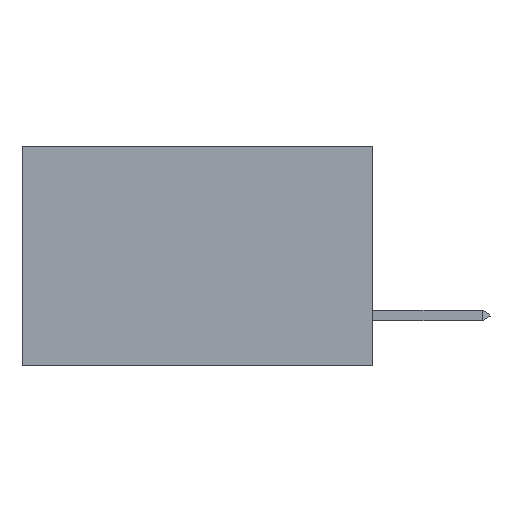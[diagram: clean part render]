
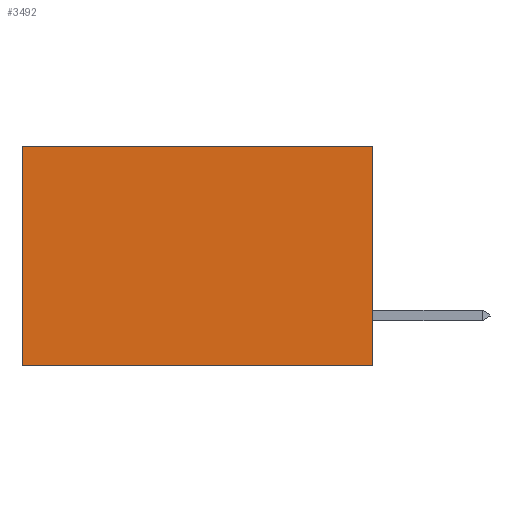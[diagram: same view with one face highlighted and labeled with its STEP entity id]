
A CAD part, left-side view. The second image highlights one B-rep face of the part: STEP entity #3492.
In plain terms, the highlighted planar face has unit normal (-1, 0, 0).
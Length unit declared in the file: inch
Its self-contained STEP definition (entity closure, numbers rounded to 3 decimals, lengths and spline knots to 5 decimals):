
#124 = ORIENTED_EDGE ( 'NONE', *, *, #6006, .F. ) ;
#918 = CARTESIAN_POINT ( 'NONE',  ( 0.277, 0.59, -0.37 ) ) ;
#1590 = CARTESIAN_POINT ( 'NONE',  ( 0.277, 0.59, -0.37 ) ) ;
#1830 = VECTOR ( 'NONE', #7440, 39.37008 ) ;
#2475 = CARTESIAN_POINT ( 'NONE',  ( 0.277, 0., 0. ) ) ;
#2851 = DIRECTION ( 'NONE',  ( 0., 0., -1. ) ) ;
#2853 = CARTESIAN_POINT ( 'NONE',  ( 0.277, 0., -0.37 ) ) ;
#3228 = LINE ( 'NONE', #1590, #7750 ) ;
#3387 = CARTESIAN_POINT ( 'NONE',  ( 0.277, 0., -0.37 ) ) ;
#3444 = PLANE ( 'NONE',  #10667 ) ;
#3492 = ADVANCED_FACE ( 'NONE', ( #8694 ), #3444, .F. ) ;
#3501 = DIRECTION ( 'NONE',  ( 0., 0., -1. ) ) ;
#3545 = DIRECTION ( 'NONE',  ( 1., 0., 0. ) ) ;
#5520 = ORIENTED_EDGE ( 'NONE', *, *, #8481, .F. ) ;
#5745 = ORIENTED_EDGE ( 'NONE', *, *, #10994, .T. ) ;
#5867 = CARTESIAN_POINT ( 'NONE',  ( 0.277, 0.59, 0. ) ) ;
#6006 = EDGE_CURVE ( 'NONE', #10157, #7099, #7083, .T. ) ;
#6203 = DIRECTION ( 'NONE',  ( 0., 0., -1. ) ) ;
#6572 = CARTESIAN_POINT ( 'NONE',  ( 0.277, 0., 0. ) ) ;
#7083 = LINE ( 'NONE', #2853, #8180 ) ;
#7099 = VERTEX_POINT ( 'NONE', #9924 ) ;
#7440 = DIRECTION ( 'NONE',  ( 0., 1., 0. ) ) ;
#7674 = CARTESIAN_POINT ( 'NONE',  ( 0.277, 0., -0.37 ) ) ;
#7750 = VECTOR ( 'NONE', #6203, 39.37008 ) ;
#7844 = VERTEX_POINT ( 'NONE', #5867 ) ;
#8180 = VECTOR ( 'NONE', #2851, 39.37008 ) ;
#8304 = VECTOR ( 'NONE', #9722, 39.37008 ) ;
#8481 = EDGE_CURVE ( 'NONE', #7099, #10109, #9129, .T. ) ;
#8608 = LINE ( 'NONE', #2475, #8304 ) ;
#8694 = FACE_OUTER_BOUND ( 'NONE', #8874, .T. ) ;
#8874 = EDGE_LOOP ( 'NONE', ( #11171, #5520, #124, #5745 ) ) ;
#9129 = LINE ( 'NONE', #7674, #1830 ) ;
#9722 = DIRECTION ( 'NONE',  ( 0., 1., 0. ) ) ;
#9924 = CARTESIAN_POINT ( 'NONE',  ( 0.277, 0., -0.37 ) ) ;
#10109 = VERTEX_POINT ( 'NONE', #918 ) ;
#10157 = VERTEX_POINT ( 'NONE', #6572 ) ;
#10667 = AXIS2_PLACEMENT_3D ( 'NONE', #3387, #3545, #3501 ) ;
#10994 = EDGE_CURVE ( 'NONE', #10157, #7844, #8608, .T. ) ;
#11057 = EDGE_CURVE ( 'NONE', #7844, #10109, #3228, .T. ) ;
#11171 = ORIENTED_EDGE ( 'NONE', *, *, #11057, .T. ) ;
